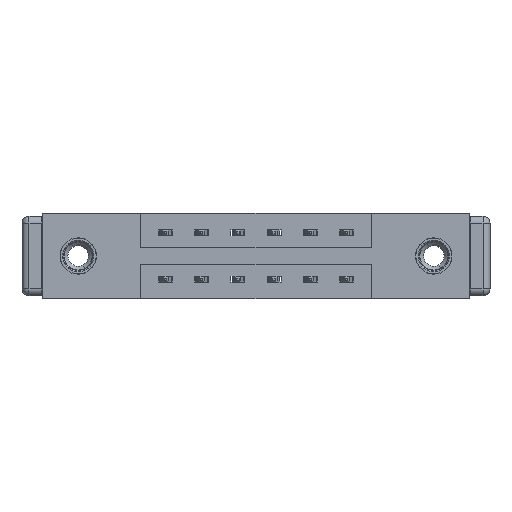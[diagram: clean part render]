
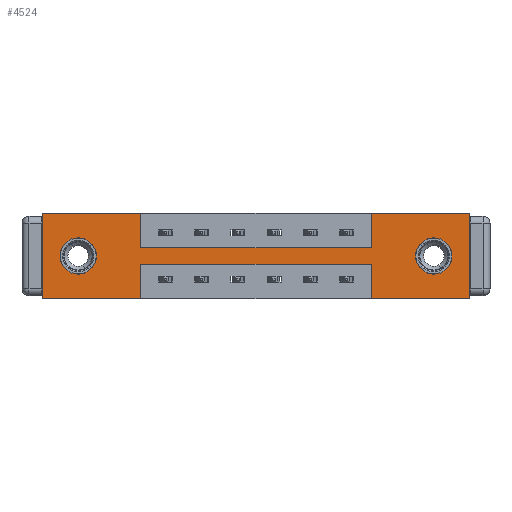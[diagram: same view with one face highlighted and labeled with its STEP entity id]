
A CAD part, front view. The second image highlights one B-rep face of the part: STEP entity #4524.
In plain terms, the highlighted planar face has unit normal (0, -1, 0).
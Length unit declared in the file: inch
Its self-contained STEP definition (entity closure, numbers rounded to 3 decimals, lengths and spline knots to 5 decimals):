
#113 = CARTESIAN_POINT ( 'NONE',  ( 1.417, 0., 0. ) ) ;
#132 = CARTESIAN_POINT ( 'NONE',  ( 0., 0., -0.37 ) ) ;
#161 = CARTESIAN_POINT ( 'NONE',  ( 1.417, 0., -0.37 ) ) ;
#349 = EDGE_CURVE ( 'NONE', #7960, #5393, #5164, .T. ) ;
#467 = CARTESIAN_POINT ( 'NONE',  ( 0., 0., 0. ) ) ;
#515 = ORIENTED_EDGE ( 'NONE', *, *, #9228, .F. ) ;
#550 = CARTESIAN_POINT ( 'NONE',  ( 0., 0., -0.37 ) ) ;
#563 = VECTOR ( 'NONE', #9985, 39.37008 ) ;
#791 = CARTESIAN_POINT ( 'NONE',  ( 0.155, 0., -0.185 ) ) ;
#830 = VECTOR ( 'NONE', #3562, 39.37008 ) ;
#867 = CARTESIAN_POINT ( 'NONE',  ( 1.417, 0., -0.22 ) ) ;
#944 = CARTESIAN_POINT ( 'NONE',  ( 1.687, 0., -0.185 ) ) ;
#967 = ORIENTED_EDGE ( 'NONE', *, *, #9918, .F. ) ;
#1011 = VECTOR ( 'NONE', #10484, 39.37008 ) ;
#1085 = DIRECTION ( 'NONE',  ( 0., -1., 0. ) ) ;
#1111 = VECTOR ( 'NONE', #7984, 39.37008 ) ;
#1199 = EDGE_CURVE ( 'NONE', #8467, #3251, #2660, .T. ) ;
#1206 = CARTESIAN_POINT ( 'NONE',  ( 0., 0., 0. ) ) ;
#1387 = FACE_OUTER_BOUND ( 'NONE', #3600, .T. ) ;
#1443 = EDGE_CURVE ( 'NONE', #7668, #4047, #6439, .T. ) ;
#1505 = EDGE_CURVE ( 'NONE', #2533, #9732, #9959, .T. ) ;
#1731 = DIRECTION ( 'NONE',  ( 0., 1., 0. ) ) ;
#1908 = ORIENTED_EDGE ( 'NONE', *, *, #2137, .F. ) ;
#2080 = CARTESIAN_POINT ( 'NONE',  ( 0.155, 0., -0.263 ) ) ;
#2137 = EDGE_CURVE ( 'NONE', #5393, #6669, #8176, .T. ) ;
#2194 = CARTESIAN_POINT ( 'NONE',  ( 0., 0., -0.37 ) ) ;
#2214 = CARTESIAN_POINT ( 'NONE',  ( 1.842, 0., 0. ) ) ;
#2279 = LINE ( 'NONE', #467, #1111 ) ;
#2366 = EDGE_CURVE ( 'NONE', #3251, #11921, #4679, .T. ) ;
#2485 = LINE ( 'NONE', #9425, #1011 ) ;
#2512 = ORIENTED_EDGE ( 'NONE', *, *, #3838, .F. ) ;
#2516 = VECTOR ( 'NONE', #10950, 39.37008 ) ;
#2533 = VERTEX_POINT ( 'NONE', #5150 ) ;
#2607 = DIRECTION ( 'NONE',  ( 0., 0., -1. ) ) ;
#2660 = LINE ( 'NONE', #10089, #2516 ) ;
#2845 = ORIENTED_EDGE ( 'NONE', *, *, #1505, .F. ) ;
#2884 = LINE ( 'NONE', #8296, #830 ) ;
#3018 = DIRECTION ( 'NONE',  ( 0., 0., -1. ) ) ;
#3033 = EDGE_CURVE ( 'NONE', #7888, #2533, #5422, .T. ) ;
#3251 = VERTEX_POINT ( 'NONE', #10706 ) ;
#3409 = DIRECTION ( 'NONE',  ( -1., 0., 0. ) ) ;
#3468 = AXIS2_PLACEMENT_3D ( 'NONE', #2194, #1085, #3018 ) ;
#3562 = DIRECTION ( 'NONE',  ( -1., 0., 0. ) ) ;
#3588 = VERTEX_POINT ( 'NONE', #1206 ) ;
#3600 = EDGE_LOOP ( 'NONE', ( #7013, #2512, #8880, #4913, #8947, #10311, #2845, #4416, #11486, #967, #515, #1908 ) ) ;
#3838 = EDGE_CURVE ( 'NONE', #11921, #7960, #2884, .T. ) ;
#3891 = CARTESIAN_POINT ( 'NONE',  ( 1.687, 0., -0.185 ) ) ;
#4009 = CARTESIAN_POINT ( 'NONE',  ( 1.687, 0., -0.107 ) ) ;
#4047 = VERTEX_POINT ( 'NONE', #7019 ) ;
#4142 = CARTESIAN_POINT ( 'NONE',  ( 0.425, 0., -0.37 ) ) ;
#4256 = EDGE_CURVE ( 'NONE', #4047, #7668, #11483, .T. ) ;
#4405 = CARTESIAN_POINT ( 'NONE',  ( 0.425, 0., -0.22 ) ) ;
#4416 = ORIENTED_EDGE ( 'NONE', *, *, #3033, .F. ) ;
#4436 = AXIS2_PLACEMENT_3D ( 'NONE', #791, #1731, #10973 ) ;
#4483 = VERTEX_POINT ( 'NONE', #2080 ) ;
#4524 = ADVANCED_FACE ( 'NONE', ( #9139, #11928, #1387 ), #10570, .T. ) ;
#4553 = ORIENTED_EDGE ( 'NONE', *, *, #4256, .T. ) ;
#4679 = LINE ( 'NONE', #161, #6267 ) ;
#4687 = VECTOR ( 'NONE', #3409, 39.37008 ) ;
#4690 = AXIS2_PLACEMENT_3D ( 'NONE', #944, #4744, #5726 ) ;
#4740 = ORIENTED_EDGE ( 'NONE', *, *, #10024, .T. ) ;
#4744 = DIRECTION ( 'NONE',  ( 0., 1., 0. ) ) ;
#4855 = DIRECTION ( 'NONE',  ( 1., 0., 0. ) ) ;
#4859 = ORIENTED_EDGE ( 'NONE', *, *, #1443, .T. ) ;
#4865 = DIRECTION ( 'NONE',  ( 0., 0., 1. ) ) ;
#4913 = ORIENTED_EDGE ( 'NONE', *, *, #1199, .F. ) ;
#5150 = CARTESIAN_POINT ( 'NONE',  ( 1.417, 0., -0.15 ) ) ;
#5164 = LINE ( 'NONE', #12073, #10132 ) ;
#5168 = CARTESIAN_POINT ( 'NONE',  ( 0., 0., 0. ) ) ;
#5295 = CARTESIAN_POINT ( 'NONE',  ( 0.425, 0., -0.15 ) ) ;
#5393 = VERTEX_POINT ( 'NONE', #4142 ) ;
#5422 = LINE ( 'NONE', #5295, #6289 ) ;
#5540 = LINE ( 'NONE', #5168, #563 ) ;
#5726 = DIRECTION ( 'NONE',  ( 0., 0., -1. ) ) ;
#5817 = CIRCLE ( 'NONE', #11717, 0.078 ) ;
#5914 = CARTESIAN_POINT ( 'NONE',  ( 0.425, 0., -0.15 ) ) ;
#5936 = CARTESIAN_POINT ( 'NONE',  ( 1.842, 0., -0.37 ) ) ;
#5981 = CARTESIAN_POINT ( 'NONE',  ( 0.155, 0., -0.185 ) ) ;
#6267 = VECTOR ( 'NONE', #4865, 39.37008 ) ;
#6289 = VECTOR ( 'NONE', #7128, 39.37008 ) ;
#6330 = AXIS2_PLACEMENT_3D ( 'NONE', #3891, #9596, #11424 ) ;
#6387 = DIRECTION ( 'NONE',  ( 0., 0., -1. ) ) ;
#6439 = CIRCLE ( 'NONE', #4690, 0.078 ) ;
#6669 = VERTEX_POINT ( 'NONE', #132 ) ;
#6819 = VERTEX_POINT ( 'NONE', #11533 ) ;
#6842 = EDGE_LOOP ( 'NONE', ( #4859, #4553 ) ) ;
#7013 = ORIENTED_EDGE ( 'NONE', *, *, #349, .F. ) ;
#7019 = CARTESIAN_POINT ( 'NONE',  ( 1.687, 0., -0.263 ) ) ;
#7128 = DIRECTION ( 'NONE',  ( 1., 0., 0. ) ) ;
#7668 = VERTEX_POINT ( 'NONE', #4009 ) ;
#7888 = VERTEX_POINT ( 'NONE', #5914 ) ;
#7960 = VERTEX_POINT ( 'NONE', #4405 ) ;
#7984 = DIRECTION ( 'NONE',  ( 0., 0., 1. ) ) ;
#8047 = VECTOR ( 'NONE', #9445, 39.37008 ) ;
#8072 = EDGE_CURVE ( 'NONE', #11432, #8467, #9736, .T. ) ;
#8176 = LINE ( 'NONE', #550, #4687 ) ;
#8296 = CARTESIAN_POINT ( 'NONE',  ( 0.425, 0., -0.22 ) ) ;
#8467 = VERTEX_POINT ( 'NONE', #5936 ) ;
#8746 = LINE ( 'NONE', #10439, #10226 ) ;
#8880 = ORIENTED_EDGE ( 'NONE', *, *, #2366, .F. ) ;
#8947 = ORIENTED_EDGE ( 'NONE', *, *, #8072, .F. ) ;
#9123 = CARTESIAN_POINT ( 'NONE',  ( 1.842, 0., 0. ) ) ;
#9139 = FACE_BOUND ( 'NONE', #6842, .T. ) ;
#9228 = EDGE_CURVE ( 'NONE', #6669, #3588, #2279, .T. ) ;
#9370 = CARTESIAN_POINT ( 'NONE',  ( 1.417, 0., 0. ) ) ;
#9425 = CARTESIAN_POINT ( 'NONE',  ( 0.425, 0., 0. ) ) ;
#9445 = DIRECTION ( 'NONE',  ( 0., 0., 1. ) ) ;
#9596 = DIRECTION ( 'NONE',  ( 0., 1., 0. ) ) ;
#9635 = CIRCLE ( 'NONE', #4436, 0.078 ) ;
#9654 = EDGE_CURVE ( 'NONE', #6819, #7888, #2485, .T. ) ;
#9693 = EDGE_CURVE ( 'NONE', #9732, #11432, #8746, .T. ) ;
#9732 = VERTEX_POINT ( 'NONE', #113 ) ;
#9736 = LINE ( 'NONE', #9123, #11187 ) ;
#9739 = DIRECTION ( 'NONE',  ( 0., 1., 0. ) ) ;
#9918 = EDGE_CURVE ( 'NONE', #3588, #6819, #5540, .T. ) ;
#9959 = LINE ( 'NONE', #9370, #8047 ) ;
#9985 = DIRECTION ( 'NONE',  ( 1., 0., 0. ) ) ;
#10024 = EDGE_CURVE ( 'NONE', #12009, #4483, #9635, .T. ) ;
#10025 = ORIENTED_EDGE ( 'NONE', *, *, #10636, .T. ) ;
#10089 = CARTESIAN_POINT ( 'NONE',  ( 0., 0., -0.37 ) ) ;
#10132 = VECTOR ( 'NONE', #6387, 39.37008 ) ;
#10226 = VECTOR ( 'NONE', #4855, 39.37008 ) ;
#10311 = ORIENTED_EDGE ( 'NONE', *, *, #9693, .F. ) ;
#10439 = CARTESIAN_POINT ( 'NONE',  ( 0., 0., 0. ) ) ;
#10484 = DIRECTION ( 'NONE',  ( 0., 0., -1. ) ) ;
#10570 = PLANE ( 'NONE',  #3468 ) ;
#10636 = EDGE_CURVE ( 'NONE', #4483, #12009, #5817, .T. ) ;
#10640 = DIRECTION ( 'NONE',  ( 0., 0., 1. ) ) ;
#10706 = CARTESIAN_POINT ( 'NONE',  ( 1.417, 0., -0.37 ) ) ;
#10950 = DIRECTION ( 'NONE',  ( -1., 0., 0. ) ) ;
#10973 = DIRECTION ( 'NONE',  ( 0., 0., 1. ) ) ;
#11187 = VECTOR ( 'NONE', #2607, 39.37008 ) ;
#11243 = CARTESIAN_POINT ( 'NONE',  ( 0.155, 0., -0.107 ) ) ;
#11314 = EDGE_LOOP ( 'NONE', ( #4740, #10025 ) ) ;
#11424 = DIRECTION ( 'NONE',  ( 0., 0., -1. ) ) ;
#11432 = VERTEX_POINT ( 'NONE', #2214 ) ;
#11483 = CIRCLE ( 'NONE', #6330, 0.078 ) ;
#11486 = ORIENTED_EDGE ( 'NONE', *, *, #9654, .F. ) ;
#11533 = CARTESIAN_POINT ( 'NONE',  ( 0.425, 0., 0. ) ) ;
#11717 = AXIS2_PLACEMENT_3D ( 'NONE', #5981, #9739, #10640 ) ;
#11921 = VERTEX_POINT ( 'NONE', #867 ) ;
#11928 = FACE_BOUND ( 'NONE', #11314, .T. ) ;
#12009 = VERTEX_POINT ( 'NONE', #11243 ) ;
#12073 = CARTESIAN_POINT ( 'NONE',  ( 0.425, 0., -0.37 ) ) ;
